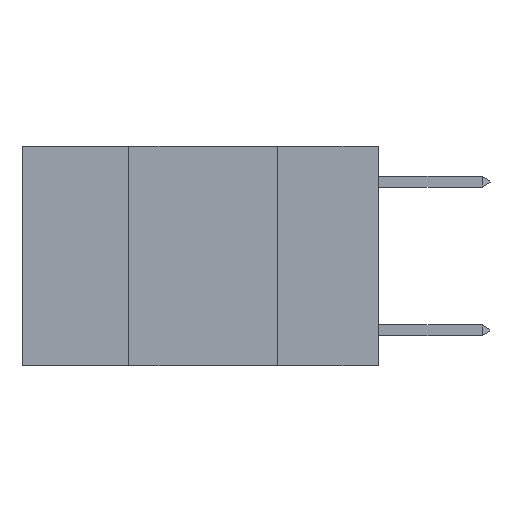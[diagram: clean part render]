
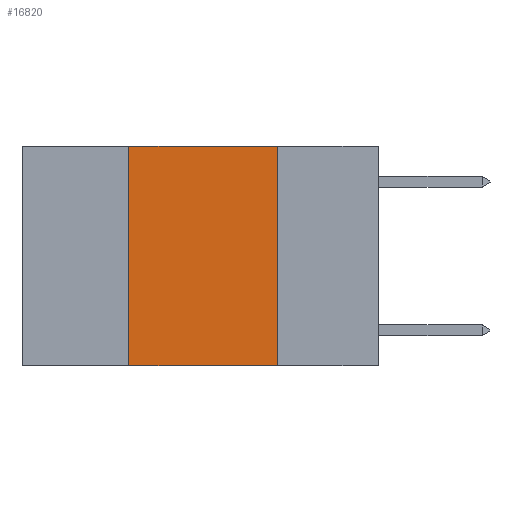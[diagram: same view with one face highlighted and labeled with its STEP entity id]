
A CAD part, left-side view. The second image highlights one B-rep face of the part: STEP entity #16820.
In plain terms, the highlighted planar face has unit normal (-1, 0, 0).
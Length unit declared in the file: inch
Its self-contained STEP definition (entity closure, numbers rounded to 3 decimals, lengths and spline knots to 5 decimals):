
#18 = LINE ( 'NONE', #11697, #4711 ) ;
#403 = FACE_OUTER_BOUND ( 'NONE', #11463, .T. ) ;
#1004 = VERTEX_POINT ( 'NONE', #16327 ) ;
#1501 = VERTEX_POINT ( 'NONE', #6712 ) ;
#1544 = DIRECTION ( 'NONE',  ( 0., -1., 0. ) ) ;
#1851 = ORIENTED_EDGE ( 'NONE', *, *, #7531, .F. ) ;
#2669 = CARTESIAN_POINT ( 'NONE',  ( 0., 0.6, 0. ) ) ;
#2855 = ORIENTED_EDGE ( 'NONE', *, *, #8115, .F. ) ;
#3323 = ORIENTED_EDGE ( 'NONE', *, *, #12393, .F. ) ;
#3370 = VECTOR ( 'NONE', #17531, 39.37008 ) ;
#3375 = ORIENTED_EDGE ( 'NONE', *, *, #15139, .T. ) ;
#4102 = DIRECTION ( 'NONE',  ( 0., 0., -1. ) ) ;
#4711 = VECTOR ( 'NONE', #1544, 39.37008 ) ;
#4955 = VECTOR ( 'NONE', #6775, 39.37008 ) ;
#4989 = VERTEX_POINT ( 'NONE', #14021 ) ;
#5418 = LINE ( 'NONE', #16781, #4955 ) ;
#5947 = AXIS2_PLACEMENT_3D ( 'NONE', #2669, #12816, #4102 ) ;
#6528 = LINE ( 'NONE', #7490, #14691 ) ;
#6712 = CARTESIAN_POINT ( 'NONE',  ( 0., 0.17, -0.37 ) ) ;
#6775 = DIRECTION ( 'NONE',  ( 0., 0., -1. ) ) ;
#7490 = CARTESIAN_POINT ( 'NONE',  ( 0., 0.6, 0. ) ) ;
#7531 = EDGE_CURVE ( 'NONE', #4989, #1004, #14491, .T. ) ;
#7584 = CARTESIAN_POINT ( 'NONE',  ( 0., 0.42, 0. ) ) ;
#8115 = EDGE_CURVE ( 'NONE', #1004, #13665, #6528, .T. ) ;
#9781 = CARTESIAN_POINT ( 'NONE',  ( 0., 0.17, 0. ) ) ;
#11463 = EDGE_LOOP ( 'NONE', ( #3323, #2855, #1851, #3375 ) ) ;
#11697 = CARTESIAN_POINT ( 'NONE',  ( 0., 0.6, -0.37 ) ) ;
#12393 = EDGE_CURVE ( 'NONE', #13665, #1501, #5418, .T. ) ;
#12816 = DIRECTION ( 'NONE',  ( 1., 0., 0. ) ) ;
#13665 = VERTEX_POINT ( 'NONE', #9781 ) ;
#14021 = CARTESIAN_POINT ( 'NONE',  ( 0., 0.42, -0.37 ) ) ;
#14491 = LINE ( 'NONE', #7584, #3370 ) ;
#14691 = VECTOR ( 'NONE', #17459, 39.37008 ) ;
#15139 = EDGE_CURVE ( 'NONE', #4989, #1501, #18, .T. ) ;
#16327 = CARTESIAN_POINT ( 'NONE',  ( 0., 0.42, 0. ) ) ;
#16781 = CARTESIAN_POINT ( 'NONE',  ( 0., 0.17, 0. ) ) ;
#16820 = ADVANCED_FACE ( 'NONE', ( #403 ), #16974, .F. ) ;
#16974 = PLANE ( 'NONE',  #5947 ) ;
#17459 = DIRECTION ( 'NONE',  ( 0., -1., 0. ) ) ;
#17531 = DIRECTION ( 'NONE',  ( 0., 0., 1. ) ) ;
